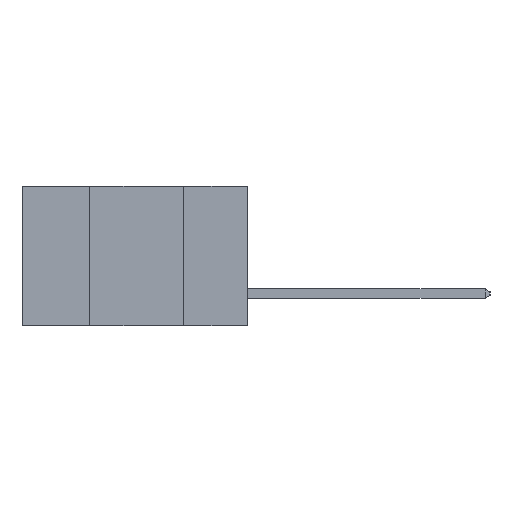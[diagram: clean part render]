
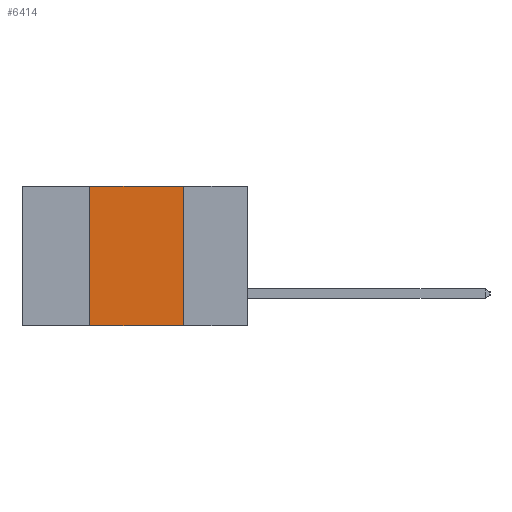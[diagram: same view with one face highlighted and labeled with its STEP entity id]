
A CAD part, left-side view. The second image highlights one B-rep face of the part: STEP entity #6414.
In plain terms, the highlighted planar face has unit normal (-1, 0, 0).
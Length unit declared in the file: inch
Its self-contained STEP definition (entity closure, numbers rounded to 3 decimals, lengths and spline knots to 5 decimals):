
#412 = CARTESIAN_POINT ( 'NONE',  ( 0., 0.42, -0.37 ) ) ;
#511 = ORIENTED_EDGE ( 'NONE', *, *, #15396, .F. ) ;
#523 = VECTOR ( 'NONE', #9271, 39.37008 ) ;
#1077 = VERTEX_POINT ( 'NONE', #13300 ) ;
#2514 = ORIENTED_EDGE ( 'NONE', *, *, #12079, .F. ) ;
#2603 = LINE ( 'NONE', #8668, #12831 ) ;
#2911 = PLANE ( 'NONE',  #3379 ) ;
#2932 = ORIENTED_EDGE ( 'NONE', *, *, #11765, .F. ) ;
#3365 = DIRECTION ( 'NONE',  ( 0., 0., -1. ) ) ;
#3379 = AXIS2_PLACEMENT_3D ( 'NONE', #3505, #3488, #3365 ) ;
#3488 = DIRECTION ( 'NONE',  ( 1., 0., 0. ) ) ;
#3505 = CARTESIAN_POINT ( 'NONE',  ( 0., 0.6, 0. ) ) ;
#4036 = VERTEX_POINT ( 'NONE', #9191 ) ;
#4648 = LINE ( 'NONE', #5510, #523 ) ;
#5510 = CARTESIAN_POINT ( 'NONE',  ( 0., 0.6, -0.37 ) ) ;
#6414 = ADVANCED_FACE ( 'NONE', ( #11990 ), #2911, .F. ) ;
#8562 = CARTESIAN_POINT ( 'NONE',  ( 0., 0.17, -0.37 ) ) ;
#8668 = CARTESIAN_POINT ( 'NONE',  ( 0., 0.6, 0. ) ) ;
#8836 = VECTOR ( 'NONE', #10873, 39.37008 ) ;
#9052 = VERTEX_POINT ( 'NONE', #8562 ) ;
#9191 = CARTESIAN_POINT ( 'NONE',  ( 0., 0.17, 0. ) ) ;
#9271 = DIRECTION ( 'NONE',  ( 0., -1., 0. ) ) ;
#9775 = ORIENTED_EDGE ( 'NONE', *, *, #10918, .T. ) ;
#9975 = VECTOR ( 'NONE', #16402, 39.37008 ) ;
#10873 = DIRECTION ( 'NONE',  ( 0., 0., 1. ) ) ;
#10918 = EDGE_CURVE ( 'NONE', #1077, #9052, #4648, .T. ) ;
#11468 = CARTESIAN_POINT ( 'NONE',  ( 0., 0.17, -0.37 ) ) ;
#11765 = EDGE_CURVE ( 'NONE', #1077, #14957, #15809, .T. ) ;
#11990 = FACE_OUTER_BOUND ( 'NONE', #16584, .T. ) ;
#12079 = EDGE_CURVE ( 'NONE', #4036, #9052, #13320, .T. ) ;
#12831 = VECTOR ( 'NONE', #16082, 39.37008 ) ;
#13300 = CARTESIAN_POINT ( 'NONE',  ( 0., 0.42, -0.37 ) ) ;
#13320 = LINE ( 'NONE', #11468, #9975 ) ;
#14957 = VERTEX_POINT ( 'NONE', #15362 ) ;
#15362 = CARTESIAN_POINT ( 'NONE',  ( 0., 0.42, 0. ) ) ;
#15396 = EDGE_CURVE ( 'NONE', #14957, #4036, #2603, .T. ) ;
#15809 = LINE ( 'NONE', #412, #8836 ) ;
#16082 = DIRECTION ( 'NONE',  ( 0., -1., 0. ) ) ;
#16402 = DIRECTION ( 'NONE',  ( 0., 0., -1. ) ) ;
#16584 = EDGE_LOOP ( 'NONE', ( #2514, #511, #2932, #9775 ) ) ;
